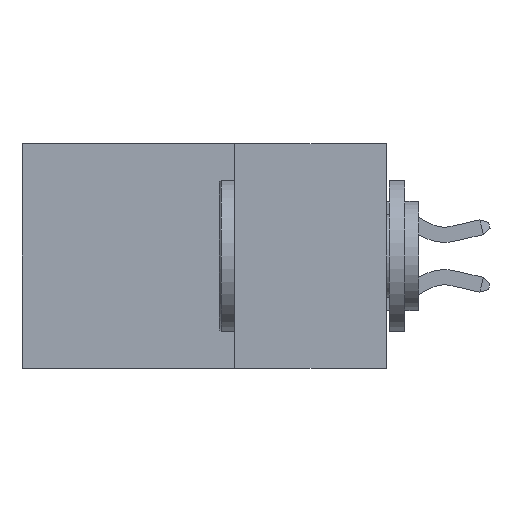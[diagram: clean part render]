
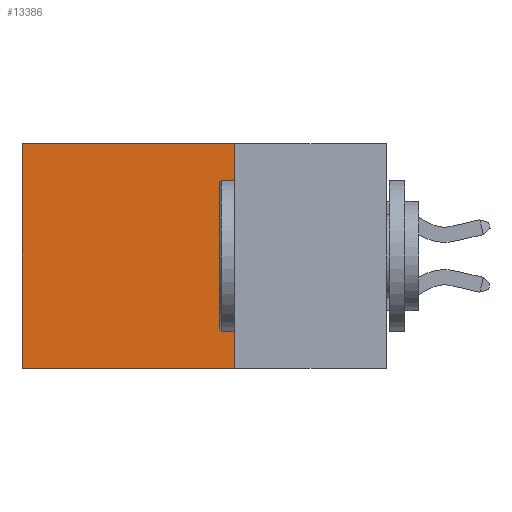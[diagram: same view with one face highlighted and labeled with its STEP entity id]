
A CAD part, left-side view. The second image highlights one B-rep face of the part: STEP entity #13386.
In plain terms, the highlighted planar face has unit normal (-1, 0, 0).
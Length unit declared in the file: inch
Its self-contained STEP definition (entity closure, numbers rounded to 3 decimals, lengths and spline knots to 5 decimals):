
#734 = VECTOR ( 'NONE', #9534, 39.37008 ) ;
#1022 = ORIENTED_EDGE ( 'NONE', *, *, #2305, .T. ) ;
#1662 = DIRECTION ( 'NONE',  ( 0., 0., -1. ) ) ;
#1707 = VECTOR ( 'NONE', #8128, 39.37008 ) ;
#1942 = DIRECTION ( 'NONE',  ( 0., 1., 0. ) ) ;
#2044 = EDGE_CURVE ( 'NONE', #7117, #2972, #12927, .T. ) ;
#2305 = EDGE_CURVE ( 'NONE', #2972, #9543, #6986, .T. ) ;
#2753 = EDGE_CURVE ( 'NONE', #12285, #9543, #10116, .T. ) ;
#2972 = VERTEX_POINT ( 'NONE', #14014 ) ;
#4635 = ORIENTED_EDGE ( 'NONE', *, *, #2044, .T. ) ;
#5135 = DIRECTION ( 'NONE',  ( 0., 0., -1. ) ) ;
#6547 = LINE ( 'NONE', #13800, #734 ) ;
#6986 = LINE ( 'NONE', #9114, #9580 ) ;
#7117 = VERTEX_POINT ( 'NONE', #9112 ) ;
#7488 = CARTESIAN_POINT ( 'NONE',  ( 0.298, 0.25, -0.37 ) ) ;
#7873 = FACE_OUTER_BOUND ( 'NONE', #13648, .T. ) ;
#8128 = DIRECTION ( 'NONE',  ( 0., 1., 0. ) ) ;
#8309 = ORIENTED_EDGE ( 'NONE', *, *, #12190, .F. ) ;
#9112 = CARTESIAN_POINT ( 'NONE',  ( 0.298, 0.25, 0. ) ) ;
#9114 = CARTESIAN_POINT ( 'NONE',  ( 0.298, 0.6, 0. ) ) ;
#9504 = PLANE ( 'NONE',  #10224 ) ;
#9534 = DIRECTION ( 'NONE',  ( 0., 0., -1. ) ) ;
#9543 = VERTEX_POINT ( 'NONE', #10215 ) ;
#9564 = CARTESIAN_POINT ( 'NONE',  ( 0.298, 0.25, -0.37 ) ) ;
#9580 = VECTOR ( 'NONE', #1662, 39.37008 ) ;
#9759 = VECTOR ( 'NONE', #1942, 39.37008 ) ;
#10116 = LINE ( 'NONE', #9564, #1707 ) ;
#10215 = CARTESIAN_POINT ( 'NONE',  ( 0.298, 0.6, -0.37 ) ) ;
#10224 = AXIS2_PLACEMENT_3D ( 'NONE', #10601, #11649, #5135 ) ;
#10601 = CARTESIAN_POINT ( 'NONE',  ( 0.298, 0.25, 0. ) ) ;
#11649 = DIRECTION ( 'NONE',  ( 1., 0., 0. ) ) ;
#12190 = EDGE_CURVE ( 'NONE', #7117, #12285, #6547, .T. ) ;
#12285 = VERTEX_POINT ( 'NONE', #7488 ) ;
#12927 = LINE ( 'NONE', #13391, #9759 ) ;
#13386 = ADVANCED_FACE ( 'NONE', ( #7873 ), #9504, .F. ) ;
#13391 = CARTESIAN_POINT ( 'NONE',  ( 0.298, 0.25, 0. ) ) ;
#13648 = EDGE_LOOP ( 'NONE', ( #1022, #13909, #8309, #4635 ) ) ;
#13800 = CARTESIAN_POINT ( 'NONE',  ( 0.298, 0.25, 0. ) ) ;
#13909 = ORIENTED_EDGE ( 'NONE', *, *, #2753, .F. ) ;
#14014 = CARTESIAN_POINT ( 'NONE',  ( 0.298, 0.6, 0. ) ) ;
